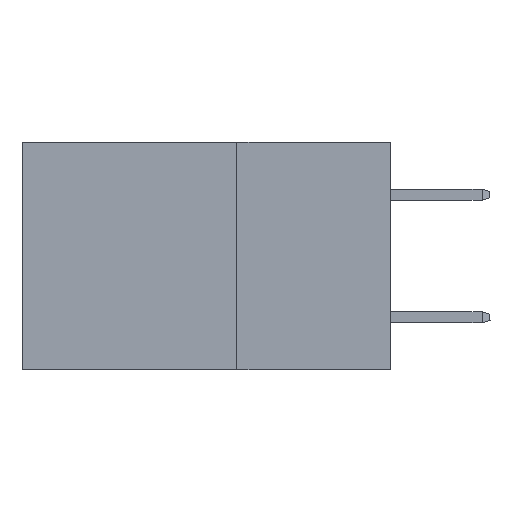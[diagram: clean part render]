
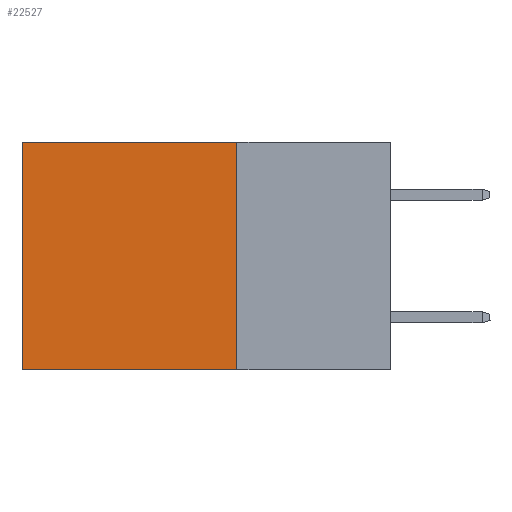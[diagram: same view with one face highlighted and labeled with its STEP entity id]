
A CAD part, left-side view. The second image highlights one B-rep face of the part: STEP entity #22527.
In plain terms, the highlighted planar face has unit normal (-1, 0, 0).
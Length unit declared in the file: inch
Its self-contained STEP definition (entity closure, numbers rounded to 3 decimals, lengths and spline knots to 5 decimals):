
#287 = EDGE_CURVE ( 'NONE', #24757, #26220, #31625, .T. ) ;
#325 = CARTESIAN_POINT ( 'NONE',  ( 0.2875, 0.6, -0.37 ) ) ;
#1597 = ORIENTED_EDGE ( 'NONE', *, *, #30226, .T. ) ;
#2358 = LINE ( 'NONE', #32722, #11189 ) ;
#2674 = ORIENTED_EDGE ( 'NONE', *, *, #287, .T. ) ;
#3214 = CARTESIAN_POINT ( 'NONE',  ( 0.2875, 0.25, -0.37 ) ) ;
#3784 = VERTEX_POINT ( 'NONE', #325 ) ;
#6144 = EDGE_LOOP ( 'NONE', ( #1597, #11825, #38703, #2674 ) ) ;
#7482 = VECTOR ( 'NONE', #21306, 39.37008 ) ;
#7899 = CARTESIAN_POINT ( 'NONE',  ( 0.2875, 0.25, 0. ) ) ;
#9385 = CARTESIAN_POINT ( 'NONE',  ( 0.2875, 0.6, 0. ) ) ;
#11189 = VECTOR ( 'NONE', #18938, 39.37008 ) ;
#11825 = ORIENTED_EDGE ( 'NONE', *, *, #37663, .F. ) ;
#12680 = VERTEX_POINT ( 'NONE', #43455 ) ;
#14218 = CARTESIAN_POINT ( 'NONE',  ( 0.2875, 0.25, 0. ) ) ;
#14285 = DIRECTION ( 'NONE',  ( 0., 0., -1. ) ) ;
#17758 = DIRECTION ( 'NONE',  ( 0., 0., -1. ) ) ;
#18938 = DIRECTION ( 'NONE',  ( 0., 0., -1. ) ) ;
#21306 = DIRECTION ( 'NONE',  ( 0., 1., 0. ) ) ;
#22527 = ADVANCED_FACE ( 'NONE', ( #43710 ), #31389, .F. ) ;
#24753 = CARTESIAN_POINT ( 'NONE',  ( 0.2875, 0.25, 0. ) ) ;
#24757 = VERTEX_POINT ( 'NONE', #7899 ) ;
#26220 = VERTEX_POINT ( 'NONE', #9385 ) ;
#26409 = LINE ( 'NONE', #3214, #7482 ) ;
#30226 = EDGE_CURVE ( 'NONE', #26220, #3784, #2358, .T. ) ;
#31389 = PLANE ( 'NONE',  #37679 ) ;
#31587 = VECTOR ( 'NONE', #41317, 39.37008 ) ;
#31625 = LINE ( 'NONE', #34575, #31587 ) ;
#32722 = CARTESIAN_POINT ( 'NONE',  ( 0.2875, 0.6, 0. ) ) ;
#34318 = VECTOR ( 'NONE', #14285, 39.37008 ) ;
#34575 = CARTESIAN_POINT ( 'NONE',  ( 0.2875, 0.25, 0. ) ) ;
#35216 = EDGE_CURVE ( 'NONE', #24757, #12680, #43240, .T. ) ;
#37663 = EDGE_CURVE ( 'NONE', #12680, #3784, #26409, .T. ) ;
#37679 = AXIS2_PLACEMENT_3D ( 'NONE', #14218, #38328, #17758 ) ;
#38328 = DIRECTION ( 'NONE',  ( 1., 0., 0. ) ) ;
#38703 = ORIENTED_EDGE ( 'NONE', *, *, #35216, .F. ) ;
#41317 = DIRECTION ( 'NONE',  ( 0., 1., 0. ) ) ;
#43240 = LINE ( 'NONE', #24753, #34318 ) ;
#43455 = CARTESIAN_POINT ( 'NONE',  ( 0.2875, 0.25, -0.37 ) ) ;
#43710 = FACE_OUTER_BOUND ( 'NONE', #6144, .T. ) ;
